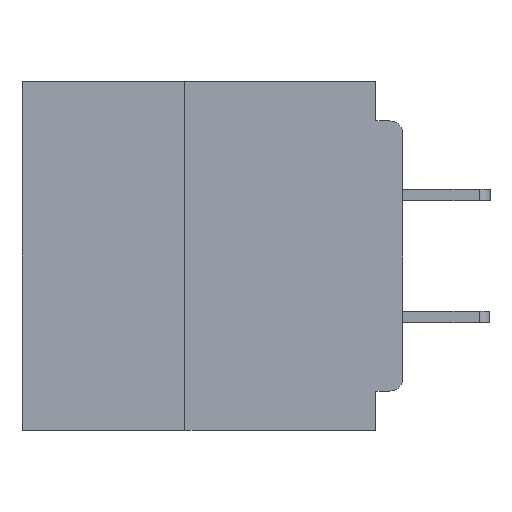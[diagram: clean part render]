
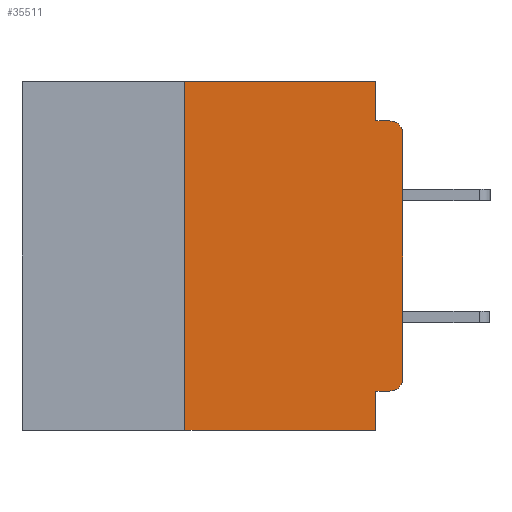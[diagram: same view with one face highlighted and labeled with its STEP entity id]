
A CAD part, left-side view. The second image highlights one B-rep face of the part: STEP entity #35511.
In plain terms, the highlighted planar face has unit normal (-1, 0, 0).
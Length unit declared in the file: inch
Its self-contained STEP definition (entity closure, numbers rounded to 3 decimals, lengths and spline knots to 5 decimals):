
#240 = EDGE_CURVE ( 'NONE', #4661, #15920, #23729, .T. ) ;
#441 = LINE ( 'NONE', #30963, #8001 ) ;
#721 = ORIENTED_EDGE ( 'NONE', *, *, #240, .F. ) ;
#1024 = ORIENTED_EDGE ( 'NONE', *, *, #22718, .T. ) ;
#1221 = FACE_OUTER_BOUND ( 'NONE', #30383, .T. ) ;
#1334 = VERTEX_POINT ( 'NONE', #1858 ) ;
#1652 = CIRCLE ( 'NONE', #30653, 0.015 ) ;
#1843 = DIRECTION ( 'NONE',  ( -1., 0., 0. ) ) ;
#1858 = CARTESIAN_POINT ( 'NONE',  ( 0., 0.031, 0. ) ) ;
#2046 = VERTEX_POINT ( 'NONE', #37398 ) ;
#2221 = VECTOR ( 'NONE', #12996, 39.37008 ) ;
#2536 = CARTESIAN_POINT ( 'NONE',  ( 0., 0., -0.34 ) ) ;
#2673 = EDGE_CURVE ( 'NONE', #27198, #15920, #18092, .T. ) ;
#2682 = VECTOR ( 'NONE', #23817, 39.37008 ) ;
#4336 = PLANE ( 'NONE',  #9461 ) ;
#4661 = VERTEX_POINT ( 'NONE', #6532 ) ;
#4739 = CARTESIAN_POINT ( 'NONE',  ( 0., 0.25, -0.4 ) ) ;
#6532 = CARTESIAN_POINT ( 'NONE',  ( 0., 0.031, -0.045 ) ) ;
#6606 = DIRECTION ( 'NONE',  ( 0., 0., 1. ) ) ;
#6998 = CARTESIAN_POINT ( 'NONE',  ( 0., 0.25, -0.4 ) ) ;
#7223 = CARTESIAN_POINT ( 'NONE',  ( 0., 0.031, -0.4 ) ) ;
#7676 = LINE ( 'NONE', #22331, #15125 ) ;
#8001 = VECTOR ( 'NONE', #40381, 39.37008 ) ;
#8989 = VERTEX_POINT ( 'NONE', #36704 ) ;
#9142 = VERTEX_POINT ( 'NONE', #2536 ) ;
#9461 = AXIS2_PLACEMENT_3D ( 'NONE', #36116, #17148, #39232 ) ;
#10438 = ORIENTED_EDGE ( 'NONE', *, *, #25649, .F. ) ;
#10455 = DIRECTION ( 'NONE',  ( 0., 0., -1. ) ) ;
#11494 = CARTESIAN_POINT ( 'NONE',  ( 0., 0., -0.355 ) ) ;
#11810 = EDGE_CURVE ( 'NONE', #11916, #40941, #19181, .T. ) ;
#11916 = VERTEX_POINT ( 'NONE', #6998 ) ;
#12458 = VECTOR ( 'NONE', #39931, 39.37008 ) ;
#12996 = DIRECTION ( 'NONE',  ( 0., -1., 0. ) ) ;
#13502 = ORIENTED_EDGE ( 'NONE', *, *, #27287, .F. ) ;
#13556 = ORIENTED_EDGE ( 'NONE', *, *, #26190, .F. ) ;
#14423 = ORIENTED_EDGE ( 'NONE', *, *, #11810, .T. ) ;
#15125 = VECTOR ( 'NONE', #6606, 39.37008 ) ;
#15920 = VERTEX_POINT ( 'NONE', #30096 ) ;
#17095 = CARTESIAN_POINT ( 'NONE',  ( 0., 0., -0.06 ) ) ;
#17148 = DIRECTION ( 'NONE',  ( 1., 0., 0. ) ) ;
#17274 = CARTESIAN_POINT ( 'NONE',  ( 0., 0.031, -0.355 ) ) ;
#17646 = LINE ( 'NONE', #4739, #2682 ) ;
#18092 = CIRCLE ( 'NONE', #24069, 0.015 ) ;
#18165 = DIRECTION ( 'NONE',  ( 0., -1., 0. ) ) ;
#19181 = LINE ( 'NONE', #28855, #2221 ) ;
#20775 = VECTOR ( 'NONE', #10455, 39.37008 ) ;
#20961 = CARTESIAN_POINT ( 'NONE',  ( 0., 0.015, -0.34 ) ) ;
#22331 = CARTESIAN_POINT ( 'NONE',  ( 0., 0., 0. ) ) ;
#22590 = DIRECTION ( 'NONE',  ( 0., 0., -1. ) ) ;
#22685 = DIRECTION ( 'NONE',  ( -1., 0., 0. ) ) ;
#22718 = EDGE_CURVE ( 'NONE', #2046, #9142, #1652, .T. ) ;
#22720 = CARTESIAN_POINT ( 'NONE',  ( 0., 0.015, -0.06 ) ) ;
#22742 = VECTOR ( 'NONE', #18165, 39.37008 ) ;
#23029 = EDGE_CURVE ( 'NONE', #9142, #27198, #7676, .T. ) ;
#23729 = LINE ( 'NONE', #38471, #22742 ) ;
#23817 = DIRECTION ( 'NONE',  ( 0., 0., 1. ) ) ;
#24069 = AXIS2_PLACEMENT_3D ( 'NONE', #22720, #22685, #22590 ) ;
#24166 = DIRECTION ( 'NONE',  ( 0., 0., -1. ) ) ;
#25231 = ORIENTED_EDGE ( 'NONE', *, *, #28864, .F. ) ;
#25649 = EDGE_CURVE ( 'NONE', #8989, #1334, #441, .T. ) ;
#26175 = CARTESIAN_POINT ( 'NONE',  ( 0., 0.031, -0.4 ) ) ;
#26190 = EDGE_CURVE ( 'NONE', #2046, #35546, #38667, .T. ) ;
#27198 = VERTEX_POINT ( 'NONE', #17095 ) ;
#27287 = EDGE_CURVE ( 'NONE', #1334, #4661, #39055, .T. ) ;
#27519 = EDGE_CURVE ( 'NONE', #35546, #40941, #29245, .T. ) ;
#28110 = CARTESIAN_POINT ( 'NONE',  ( 0., 0.031, 0. ) ) ;
#28855 = CARTESIAN_POINT ( 'NONE',  ( 0., 0.437, -0.4 ) ) ;
#28864 = EDGE_CURVE ( 'NONE', #11916, #8989, #17646, .T. ) ;
#29245 = LINE ( 'NONE', #7223, #20775 ) ;
#29768 = VECTOR ( 'NONE', #37296, 39.37008 ) ;
#30096 = CARTESIAN_POINT ( 'NONE',  ( 0., 0.015, -0.045 ) ) ;
#30383 = EDGE_LOOP ( 'NONE', ( #31728, #39117, #721, #13502, #10438, #25231, #14423, #34982, #13556, #1024 ) ) ;
#30653 = AXIS2_PLACEMENT_3D ( 'NONE', #20961, #1843, #24166 ) ;
#30963 = CARTESIAN_POINT ( 'NONE',  ( 0., 0.437, 0. ) ) ;
#31728 = ORIENTED_EDGE ( 'NONE', *, *, #23029, .T. ) ;
#34982 = ORIENTED_EDGE ( 'NONE', *, *, #27519, .F. ) ;
#35511 = ADVANCED_FACE ( 'NONE', ( #1221 ), #4336, .F. ) ;
#35546 = VERTEX_POINT ( 'NONE', #17274 ) ;
#36116 = CARTESIAN_POINT ( 'NONE',  ( 0., 0.437, 0. ) ) ;
#36704 = CARTESIAN_POINT ( 'NONE',  ( 0., 0.25, 0. ) ) ;
#37296 = DIRECTION ( 'NONE',  ( 0., 0., -1. ) ) ;
#37398 = CARTESIAN_POINT ( 'NONE',  ( 0., 0.015, -0.355 ) ) ;
#38471 = CARTESIAN_POINT ( 'NONE',  ( 0., 0., -0.045 ) ) ;
#38667 = LINE ( 'NONE', #11494, #12458 ) ;
#39055 = LINE ( 'NONE', #28110, #29768 ) ;
#39117 = ORIENTED_EDGE ( 'NONE', *, *, #2673, .T. ) ;
#39232 = DIRECTION ( 'NONE',  ( 0., 0., -1. ) ) ;
#39931 = DIRECTION ( 'NONE',  ( 0., 1., 0. ) ) ;
#40381 = DIRECTION ( 'NONE',  ( 0., -1., 0. ) ) ;
#40941 = VERTEX_POINT ( 'NONE', #26175 ) ;
